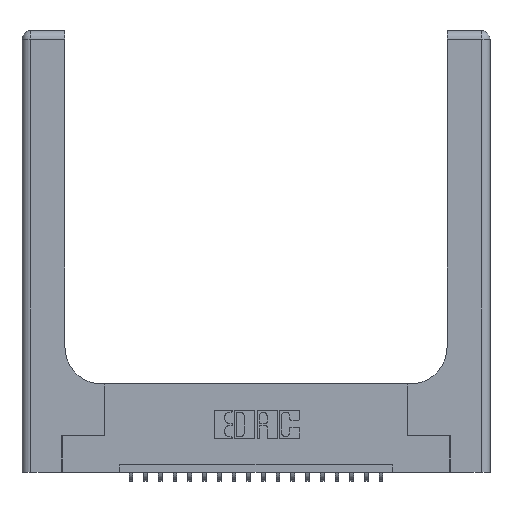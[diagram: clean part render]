
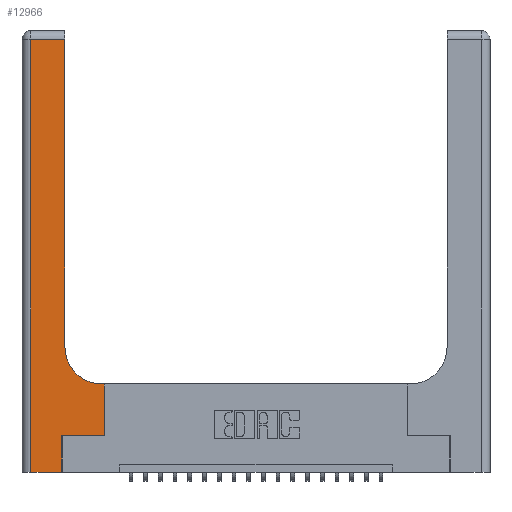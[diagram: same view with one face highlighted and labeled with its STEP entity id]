
A CAD part, top view. The second image highlights one B-rep face of the part: STEP entity #12966.
In plain terms, the highlighted planar face has unit normal (0, 0, 1).
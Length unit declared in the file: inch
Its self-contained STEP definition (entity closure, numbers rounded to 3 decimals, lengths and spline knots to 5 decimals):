
#784 = ORIENTED_EDGE ( 'NONE', *, *, #4791, .T. ) ;
#977 = DIRECTION ( 'NONE',  ( -1., 0., 0. ) ) ;
#1080 = DIRECTION ( 'NONE',  ( 0., -1., 0. ) ) ;
#1136 = DIRECTION ( 'NONE',  ( 0., 1., 0. ) ) ;
#1203 = CARTESIAN_POINT ( 'NONE',  ( 0.2915, 2.94, 0.37 ) ) ;
#1606 = VECTOR ( 'NONE', #13033, 39.37008 ) ;
#1901 = VECTOR ( 'NONE', #977, 39.37008 ) ;
#2493 = VERTEX_POINT ( 'NONE', #18223 ) ;
#2508 = VECTOR ( 'NONE', #13456, 39.37008 ) ;
#2626 = DIRECTION ( 'NONE',  ( 1., 0., 0. ) ) ;
#2730 = ORIENTED_EDGE ( 'NONE', *, *, #18920, .T. ) ;
#3312 = DIRECTION ( 'NONE',  ( 0., 0., -1. ) ) ;
#3460 = VERTEX_POINT ( 'NONE', #1203 ) ;
#3742 = VERTEX_POINT ( 'NONE', #21195 ) ;
#4219 = VERTEX_POINT ( 'NONE', #20383 ) ;
#4618 = LINE ( 'NONE', #16345, #18165 ) ;
#4625 = EDGE_CURVE ( 'NONE', #2493, #4219, #13591, .T. ) ;
#4718 = CARTESIAN_POINT ( 'NONE',  ( 0., 3., 0.37 ) ) ;
#4791 = EDGE_CURVE ( 'NONE', #4933, #16392, #15442, .T. ) ;
#4933 = VERTEX_POINT ( 'NONE', #21570 ) ;
#5342 = LINE ( 'NONE', #12446, #17551 ) ;
#5371 = VECTOR ( 'NONE', #17737, 39.37008 ) ;
#5914 = VERTEX_POINT ( 'NONE', #11012 ) ;
#5965 = CARTESIAN_POINT ( 'NONE',  ( 0.5415, 0.85, 0.37 ) ) ;
#6417 = VECTOR ( 'NONE', #20271, 39.37008 ) ;
#7160 = LINE ( 'NONE', #19765, #1606 ) ;
#7176 = ORIENTED_EDGE ( 'NONE', *, *, #17254, .T. ) ;
#7272 = ORIENTED_EDGE ( 'NONE', *, *, #4625, .T. ) ;
#7917 = VERTEX_POINT ( 'NONE', #20005 ) ;
#8086 = DIRECTION ( 'NONE',  ( -1., 0., 0. ) ) ;
#8115 = CIRCLE ( 'NONE', #15380, 0.25 ) ;
#8766 = ORIENTED_EDGE ( 'NONE', *, *, #17095, .T. ) ;
#9225 = ORIENTED_EDGE ( 'NONE', *, *, #20422, .T. ) ;
#9324 = AXIS2_PLACEMENT_3D ( 'NONE', #4718, #3312, #20255 ) ;
#11012 = CARTESIAN_POINT ( 'NONE',  ( 0.06, 0., 0.37 ) ) ;
#11448 = CARTESIAN_POINT ( 'NONE',  ( 0., 2.94, 0.37 ) ) ;
#12301 = VECTOR ( 'NONE', #8086, 39.37008 ) ;
#12304 = CARTESIAN_POINT ( 'NONE',  ( 0.2915, 0.6, 0.37 ) ) ;
#12446 = CARTESIAN_POINT ( 'NONE',  ( 0.06, 3., 0.37 ) ) ;
#12798 = LINE ( 'NONE', #19306, #5371 ) ;
#12966 = ADVANCED_FACE ( 'NONE', ( #20927 ), #13225, .F. ) ;
#13033 = DIRECTION ( 'NONE',  ( 0., 1., 0. ) ) ;
#13225 = PLANE ( 'NONE',  #9324 ) ;
#13456 = DIRECTION ( 'NONE',  ( 1., 0., 0. ) ) ;
#13591 = LINE ( 'NONE', #12304, #1901 ) ;
#14566 = EDGE_CURVE ( 'NONE', #3742, #5914, #5342, .T. ) ;
#15380 = AXIS2_PLACEMENT_3D ( 'NONE', #5965, #19561, #2626 ) ;
#15442 = LINE ( 'NONE', #20350, #6417 ) ;
#15532 = CARTESIAN_POINT ( 'NONE',  ( 0.5585, 0.25, 0.37 ) ) ;
#15740 = EDGE_CURVE ( 'NONE', #4219, #7917, #8115, .T. ) ;
#15945 = EDGE_CURVE ( 'NONE', #5914, #4933, #17384, .T. ) ;
#16345 = CARTESIAN_POINT ( 'NONE',  ( 0.2915, 3., 0.37 ) ) ;
#16357 = ORIENTED_EDGE ( 'NONE', *, *, #14566, .T. ) ;
#16392 = VERTEX_POINT ( 'NONE', #16713 ) ;
#16556 = ORIENTED_EDGE ( 'NONE', *, *, #15740, .T. ) ;
#16713 = CARTESIAN_POINT ( 'NONE',  ( 0.269, 0.25, 0.37 ) ) ;
#17095 = EDGE_CURVE ( 'NONE', #16392, #19119, #12798, .T. ) ;
#17254 = EDGE_CURVE ( 'NONE', #3460, #3742, #20548, .T. ) ;
#17384 = LINE ( 'NONE', #21985, #2508 ) ;
#17551 = VECTOR ( 'NONE', #1080, 39.37008 ) ;
#17737 = DIRECTION ( 'NONE',  ( 1., 0., 0. ) ) ;
#18165 = VECTOR ( 'NONE', #1136, 39.37008 ) ;
#18223 = CARTESIAN_POINT ( 'NONE',  ( 0.5585, 0.6, 0.37 ) ) ;
#18920 = EDGE_CURVE ( 'NONE', #19119, #2493, #7160, .T. ) ;
#19119 = VERTEX_POINT ( 'NONE', #15532 ) ;
#19306 = CARTESIAN_POINT ( 'NONE',  ( 0.269, 0.25, 0.37 ) ) ;
#19561 = DIRECTION ( 'NONE',  ( 0., 0., -1. ) ) ;
#19765 = CARTESIAN_POINT ( 'NONE',  ( 0.5585, 0.25, 0.37 ) ) ;
#20005 = CARTESIAN_POINT ( 'NONE',  ( 0.2915, 0.85, 0.37 ) ) ;
#20255 = DIRECTION ( 'NONE',  ( -1., 0., 0. ) ) ;
#20271 = DIRECTION ( 'NONE',  ( 0., 1., 0. ) ) ;
#20350 = CARTESIAN_POINT ( 'NONE',  ( 0.269, 0., 0.37 ) ) ;
#20383 = CARTESIAN_POINT ( 'NONE',  ( 0.5415, 0.6, 0.37 ) ) ;
#20422 = EDGE_CURVE ( 'NONE', #7917, #3460, #4618, .T. ) ;
#20548 = LINE ( 'NONE', #11448, #12301 ) ;
#20806 = ORIENTED_EDGE ( 'NONE', *, *, #15945, .T. ) ;
#20927 = FACE_OUTER_BOUND ( 'NONE', #21815, .T. ) ;
#21195 = CARTESIAN_POINT ( 'NONE',  ( 0.06, 2.94, 0.37 ) ) ;
#21570 = CARTESIAN_POINT ( 'NONE',  ( 0.269, 0., 0.37 ) ) ;
#21815 = EDGE_LOOP ( 'NONE', ( #9225, #7176, #16357, #20806, #784, #8766, #2730, #7272, #16556 ) ) ;
#21985 = CARTESIAN_POINT ( 'NONE',  ( 0., 0., 0.37 ) ) ;
